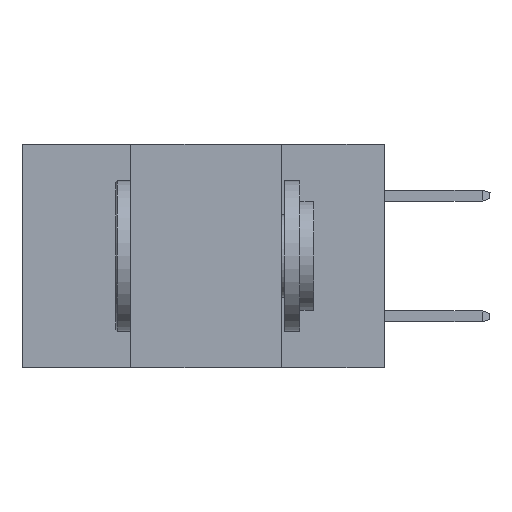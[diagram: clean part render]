
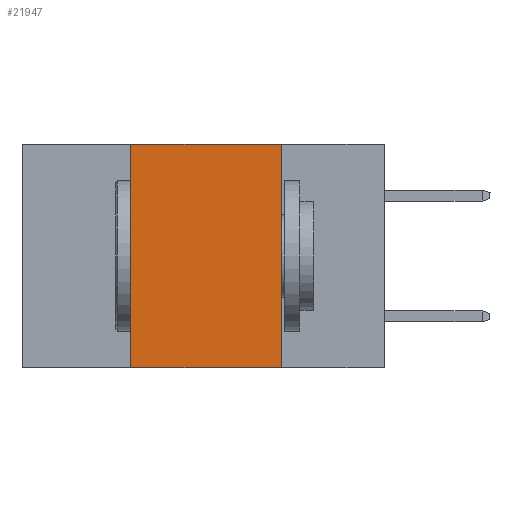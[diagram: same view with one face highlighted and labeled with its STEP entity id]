
A CAD part, left-side view. The second image highlights one B-rep face of the part: STEP entity #21947.
In plain terms, the highlighted planar face has unit normal (-1, 0, 0).
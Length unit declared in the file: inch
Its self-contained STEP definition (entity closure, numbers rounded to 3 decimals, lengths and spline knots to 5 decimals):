
#147 = CARTESIAN_POINT ( 'NONE',  ( 0., 0.6, 0. ) ) ;
#1215 = ORIENTED_EDGE ( 'NONE', *, *, #4139, .F. ) ;
#1295 = DIRECTION ( 'NONE',  ( 0., 0., -1. ) ) ;
#2664 = CARTESIAN_POINT ( 'NONE',  ( 0., 0.42, -0.37 ) ) ;
#2705 = DIRECTION ( 'NONE',  ( 0., 0., 1. ) ) ;
#2957 = CARTESIAN_POINT ( 'NONE',  ( 0., 0.42, 0. ) ) ;
#3912 = DIRECTION ( 'NONE',  ( 1., 0., 0. ) ) ;
#4139 = EDGE_CURVE ( 'NONE', #22017, #11248, #24365, .T. ) ;
#6157 = CARTESIAN_POINT ( 'NONE',  ( 0., 0.6, -0.37 ) ) ;
#6387 = CARTESIAN_POINT ( 'NONE',  ( 0., 0.42, 0. ) ) ;
#6440 = ORIENTED_EDGE ( 'NONE', *, *, #21252, .F. ) ;
#6532 = ORIENTED_EDGE ( 'NONE', *, *, #7935, .T. ) ;
#6962 = CARTESIAN_POINT ( 'NONE',  ( 0., 0.6, 0. ) ) ;
#7896 = CARTESIAN_POINT ( 'NONE',  ( 0., 0.17, -0.37 ) ) ;
#7935 = EDGE_CURVE ( 'NONE', #22017, #16936, #20023, .T. ) ;
#9217 = VECTOR ( 'NONE', #12360, 39.37008 ) ;
#10501 = EDGE_CURVE ( 'NONE', #17517, #16936, #15252, .T. ) ;
#11248 = VERTEX_POINT ( 'NONE', #6387 ) ;
#12223 = PLANE ( 'NONE',  #16095 ) ;
#12360 = DIRECTION ( 'NONE',  ( 0., -1., 0. ) ) ;
#13828 = CARTESIAN_POINT ( 'NONE',  ( 0., 0.17, 0. ) ) ;
#14303 = DIRECTION ( 'NONE',  ( 0., 0., -1. ) ) ;
#14526 = LINE ( 'NONE', #6962, #18985 ) ;
#14970 = ORIENTED_EDGE ( 'NONE', *, *, #10501, .F. ) ;
#15166 = EDGE_LOOP ( 'NONE', ( #14970, #6440, #1215, #6532 ) ) ;
#15252 = LINE ( 'NONE', #13828, #23473 ) ;
#16095 = AXIS2_PLACEMENT_3D ( 'NONE', #147, #3912, #14303 ) ;
#16936 = VERTEX_POINT ( 'NONE', #7896 ) ;
#17517 = VERTEX_POINT ( 'NONE', #23851 ) ;
#18985 = VECTOR ( 'NONE', #25063, 39.37008 ) ;
#19019 = VECTOR ( 'NONE', #2705, 39.37008 ) ;
#20023 = LINE ( 'NONE', #6157, #9217 ) ;
#21252 = EDGE_CURVE ( 'NONE', #11248, #17517, #14526, .T. ) ;
#21947 = ADVANCED_FACE ( 'NONE', ( #22396 ), #12223, .F. ) ;
#22017 = VERTEX_POINT ( 'NONE', #2664 ) ;
#22396 = FACE_OUTER_BOUND ( 'NONE', #15166, .T. ) ;
#23473 = VECTOR ( 'NONE', #1295, 39.37008 ) ;
#23851 = CARTESIAN_POINT ( 'NONE',  ( 0., 0.17, 0. ) ) ;
#24365 = LINE ( 'NONE', #2957, #19019 ) ;
#25063 = DIRECTION ( 'NONE',  ( 0., -1., 0. ) ) ;
